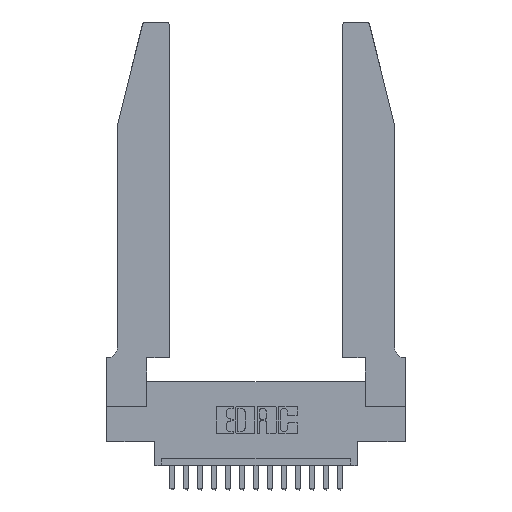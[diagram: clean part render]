
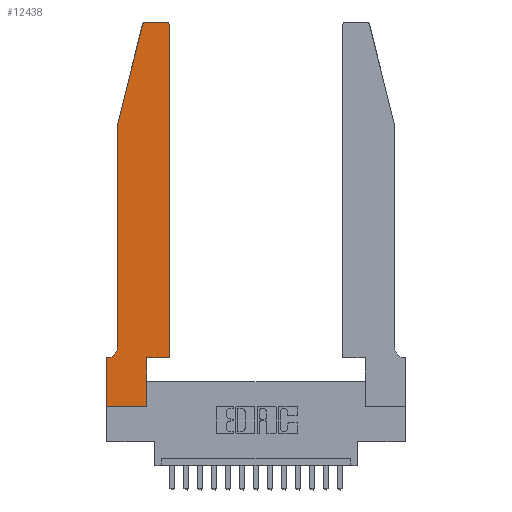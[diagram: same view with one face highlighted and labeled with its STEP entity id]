
A CAD part, top view. The second image highlights one B-rep face of the part: STEP entity #12438.
In plain terms, the highlighted planar face has unit normal (0, 0, 1).
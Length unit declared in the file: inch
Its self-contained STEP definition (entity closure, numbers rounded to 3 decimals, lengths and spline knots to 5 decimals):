
#17 = ORIENTED_EDGE ( 'NONE', *, *, #16861, .T. ) ;
#499 = VERTEX_POINT ( 'NONE', #9638 ) ;
#717 = ORIENTED_EDGE ( 'NONE', *, *, #9147, .T. ) ;
#772 = CARTESIAN_POINT ( 'NONE',  ( 0.0055, 0.35, 0.37 ) ) ;
#867 = LINE ( 'NONE', #15262, #14617 ) ;
#1013 = LINE ( 'NONE', #12189, #13431 ) ;
#1458 = ORIENTED_EDGE ( 'NONE', *, *, #13365, .T. ) ;
#1472 = VECTOR ( 'NONE', #9612, 39.37008 ) ;
#1501 = VERTEX_POINT ( 'NONE', #12512 ) ;
#1744 = EDGE_CURVE ( 'NONE', #14608, #1501, #12470, .T. ) ;
#1812 = CARTESIAN_POINT ( 'NONE',  ( 0.0755, 0.35, 0.37 ) ) ;
#1835 = CARTESIAN_POINT ( 'NONE',  ( 0., 0., 0.37 ) ) ;
#2456 = DIRECTION ( 'NONE',  ( 0., 0., 1. ) ) ;
#2471 = DIRECTION ( 'NONE',  ( 1., 0., 0. ) ) ;
#2592 = LINE ( 'NONE', #6521, #1472 ) ;
#3266 = ORIENTED_EDGE ( 'NONE', *, *, #6695, .T. ) ;
#4131 = ORIENTED_EDGE ( 'NONE', *, *, #13020, .T. ) ;
#4827 = ORIENTED_EDGE ( 'NONE', *, *, #7052, .T. ) ;
#4870 = ORIENTED_EDGE ( 'NONE', *, *, #12488, .T. ) ;
#5159 = CARTESIAN_POINT ( 'NONE',  ( 0.4505, 2.72, 0.37 ) ) ;
#5218 = PLANE ( 'NONE',  #8936 ) ;
#5248 = CARTESIAN_POINT ( 'NONE',  ( 0., 0., 0.37 ) ) ;
#5401 = VERTEX_POINT ( 'NONE', #15329 ) ;
#5516 = AXIS2_PLACEMENT_3D ( 'NONE', #6761, #2456, #9533 ) ;
#5519 = LINE ( 'NONE', #5248, #8947 ) ;
#5741 = VERTEX_POINT ( 'NONE', #5159 ) ;
#5983 = DIRECTION ( 'NONE',  ( 0., 0., 1. ) ) ;
#6172 = CARTESIAN_POINT ( 'NONE',  ( 0.284, 2.72, 0.37 ) ) ;
#6392 = VECTOR ( 'NONE', #12010, 39.37008 ) ;
#6521 = CARTESIAN_POINT ( 'NONE',  ( 0.4505, 0.35, 0.37 ) ) ;
#6655 = DIRECTION ( 'NONE',  ( 0., 0., 1. ) ) ;
#6673 = CARTESIAN_POINT ( 'NONE',  ( 0.0755, 2., 0.37 ) ) ;
#6695 = EDGE_CURVE ( 'NONE', #6835, #5741, #2592, .T. ) ;
#6761 = CARTESIAN_POINT ( 'NONE',  ( 0.4205, 2.72, 0.37 ) ) ;
#6835 = VERTEX_POINT ( 'NONE', #17224 ) ;
#7052 = EDGE_CURVE ( 'NONE', #13620, #5401, #16072, .T. ) ;
#7379 = VECTOR ( 'NONE', #11015, 39.37008 ) ;
#7387 = DIRECTION ( 'NONE',  ( 0., 0., -1. ) ) ;
#7679 = DIRECTION ( 'NONE',  ( 1., 0., 0. ) ) ;
#7753 = CIRCLE ( 'NONE', #5516, 0.03 ) ;
#7913 = AXIS2_PLACEMENT_3D ( 'NONE', #8808, #7387, #14595 ) ;
#7969 = CARTESIAN_POINT ( 'NONE',  ( 0.284, 2.75, 0.37 ) ) ;
#8101 = ORIENTED_EDGE ( 'NONE', *, *, #13405, .T. ) ;
#8246 = VERTEX_POINT ( 'NONE', #6673 ) ;
#8273 = CARTESIAN_POINT ( 'NONE',  ( 0., 0.35, 0.37 ) ) ;
#8283 = VERTEX_POINT ( 'NONE', #18313 ) ;
#8305 = ORIENTED_EDGE ( 'NONE', *, *, #14091, .T. ) ;
#8608 = CIRCLE ( 'NONE', #7913, 0.07 ) ;
#8808 = CARTESIAN_POINT ( 'NONE',  ( 0.0055, 0.42, 0.37 ) ) ;
#8936 = AXIS2_PLACEMENT_3D ( 'NONE', #8273, #6655, #2471 ) ;
#8947 = VECTOR ( 'NONE', #11236, 39.37008 ) ;
#9066 = LINE ( 'NONE', #18465, #7379 ) ;
#9147 = EDGE_CURVE ( 'NONE', #10592, #13620, #8608, .T. ) ;
#9402 = CARTESIAN_POINT ( 'NONE',  ( 0.0755, 0.42, 0.37 ) ) ;
#9533 = DIRECTION ( 'NONE',  ( 1., 0., 0. ) ) ;
#9612 = DIRECTION ( 'NONE',  ( 0., 1., 0. ) ) ;
#9638 = CARTESIAN_POINT ( 'NONE',  ( 0.4205, 2.75, 0.37 ) ) ;
#9764 = DIRECTION ( 'NONE',  ( 0., -1., 0. ) ) ;
#9959 = ORIENTED_EDGE ( 'NONE', *, *, #11565, .T. ) ;
#10328 = VERTEX_POINT ( 'NONE', #18593 ) ;
#10592 = VERTEX_POINT ( 'NONE', #9402 ) ;
#10999 = DIRECTION ( 'NONE',  ( -1., 0., 0. ) ) ;
#11015 = DIRECTION ( 'NONE',  ( 0., 1., 0. ) ) ;
#11236 = DIRECTION ( 'NONE',  ( 0., -1., 0. ) ) ;
#11565 = EDGE_CURVE ( 'NONE', #8246, #10592, #867, .T. ) ;
#12010 = DIRECTION ( 'NONE',  ( -0.239, -0.971, 0. ) ) ;
#12189 = CARTESIAN_POINT ( 'NONE',  ( 0.2605, 2.75, 0.37 ) ) ;
#12288 = VECTOR ( 'NONE', #10999, 39.37008 ) ;
#12438 = ADVANCED_FACE ( 'NONE', ( #14358 ), #5218, .T. ) ;
#12455 = LINE ( 'NONE', #1835, #13356 ) ;
#12470 = CIRCLE ( 'NONE', #16162, 0.03 ) ;
#12488 = EDGE_CURVE ( 'NONE', #10328, #6835, #16607, .T. ) ;
#12512 = CARTESIAN_POINT ( 'NONE',  ( 0.25487, 2.72718, 0.37 ) ) ;
#13020 = EDGE_CURVE ( 'NONE', #5401, #17523, #5519, .T. ) ;
#13356 = VECTOR ( 'NONE', #7679, 39.37008 ) ;
#13365 = EDGE_CURVE ( 'NONE', #1501, #8246, #14534, .T. ) ;
#13405 = EDGE_CURVE ( 'NONE', #499, #14608, #1013, .T. ) ;
#13431 = VECTOR ( 'NONE', #14827, 39.37008 ) ;
#13620 = VERTEX_POINT ( 'NONE', #772 ) ;
#13970 = ORIENTED_EDGE ( 'NONE', *, *, #16520, .T. ) ;
#14091 = EDGE_CURVE ( 'NONE', #5741, #499, #7753, .T. ) ;
#14358 = FACE_OUTER_BOUND ( 'NONE', #15881, .T. ) ;
#14534 = LINE ( 'NONE', #16258, #6392 ) ;
#14595 = DIRECTION ( 'NONE',  ( -1., 0., 0. ) ) ;
#14608 = VERTEX_POINT ( 'NONE', #7969 ) ;
#14617 = VECTOR ( 'NONE', #9764, 39.37008 ) ;
#14768 = ORIENTED_EDGE ( 'NONE', *, *, #1744, .T. ) ;
#14827 = DIRECTION ( 'NONE',  ( -1., 0., 0. ) ) ;
#15262 = CARTESIAN_POINT ( 'NONE',  ( 0.0755, 2., 0.37 ) ) ;
#15329 = CARTESIAN_POINT ( 'NONE',  ( 0., 0.35, 0.37 ) ) ;
#15881 = EDGE_LOOP ( 'NONE', ( #8101, #14768, #1458, #9959, #717, #4827, #4131, #13970, #17, #4870, #3266, #8305 ) ) ;
#16072 = LINE ( 'NONE', #1812, #12288 ) ;
#16162 = AXIS2_PLACEMENT_3D ( 'NONE', #6172, #5983, #16326 ) ;
#16258 = CARTESIAN_POINT ( 'NONE',  ( 0.0755, 2., 0.37 ) ) ;
#16326 = DIRECTION ( 'NONE',  ( 1., 0., 0. ) ) ;
#16520 = EDGE_CURVE ( 'NONE', #17523, #8283, #12455, .T. ) ;
#16607 = LINE ( 'NONE', #18294, #17300 ) ;
#16618 = CARTESIAN_POINT ( 'NONE',  ( 0., 0., 0.37 ) ) ;
#16861 = EDGE_CURVE ( 'NONE', #8283, #10328, #9066, .T. ) ;
#17224 = CARTESIAN_POINT ( 'NONE',  ( 0.4505, 0.35, 0.37 ) ) ;
#17300 = VECTOR ( 'NONE', #18601, 39.37008 ) ;
#17523 = VERTEX_POINT ( 'NONE', #16618 ) ;
#18294 = CARTESIAN_POINT ( 'NONE',  ( 0.4505, 0.35, 0.37 ) ) ;
#18313 = CARTESIAN_POINT ( 'NONE',  ( 0.2865, 0., 0.37 ) ) ;
#18465 = CARTESIAN_POINT ( 'NONE',  ( 0.2865, 0.35, 0.37 ) ) ;
#18593 = CARTESIAN_POINT ( 'NONE',  ( 0.2865, 0.35, 0.37 ) ) ;
#18601 = DIRECTION ( 'NONE',  ( 1., 0., 0. ) ) ;
